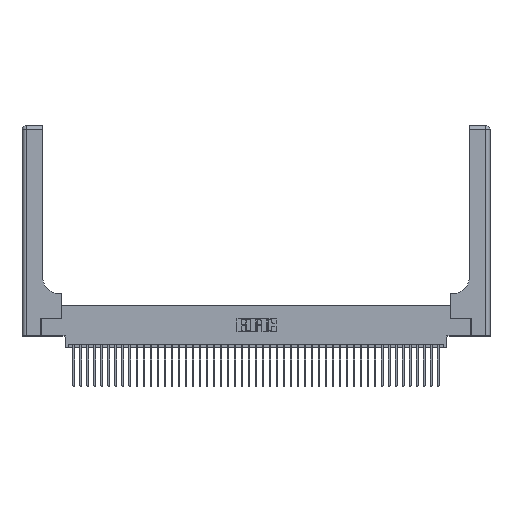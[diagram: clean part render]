
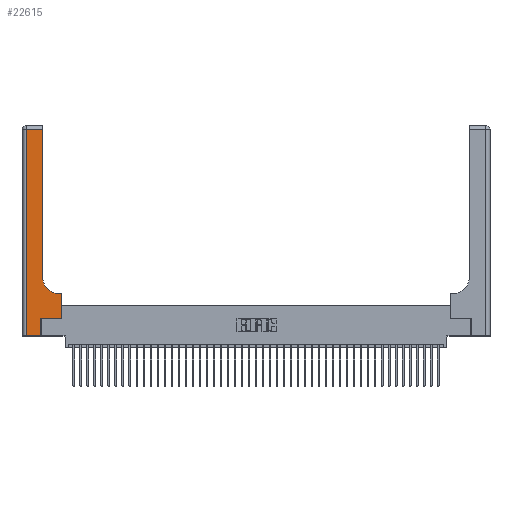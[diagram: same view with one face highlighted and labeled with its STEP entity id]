
A CAD part, top view. The second image highlights one B-rep face of the part: STEP entity #22615.
In plain terms, the highlighted planar face has unit normal (0, 0, 1).
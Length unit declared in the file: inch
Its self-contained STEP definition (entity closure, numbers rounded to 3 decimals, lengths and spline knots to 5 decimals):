
#1185 = VECTOR ( 'NONE', #26583, 39.37008 ) ;
#1284 = DIRECTION ( 'NONE',  ( 0., 1., 0. ) ) ;
#3033 = EDGE_LOOP ( 'NONE', ( #35671, #35020, #24982, #42316, #6401, #29921, #36176, #27049, #35757 ) ) ;
#3114 = VERTEX_POINT ( 'NONE', #22190 ) ;
#5375 = VECTOR ( 'NONE', #28450, 39.37008 ) ;
#5903 = VECTOR ( 'NONE', #1284, 39.37008 ) ;
#6401 = ORIENTED_EDGE ( 'NONE', *, *, #17791, .T. ) ;
#8280 = CARTESIAN_POINT ( 'NONE',  ( 0.5415, 0.6, 0.37 ) ) ;
#8372 = CARTESIAN_POINT ( 'NONE',  ( 0.2915, 0.6, 0.37 ) ) ;
#8870 = DIRECTION ( 'NONE',  ( 1., 0., 0. ) ) ;
#9039 = EDGE_CURVE ( 'NONE', #22875, #18721, #40002, .T. ) ;
#11078 = DIRECTION ( 'NONE',  ( 0., 0., -1. ) ) ;
#11527 = VERTEX_POINT ( 'NONE', #27741 ) ;
#11556 = CARTESIAN_POINT ( 'NONE',  ( 0.269, 0.25, 0.37 ) ) ;
#12474 = CARTESIAN_POINT ( 'NONE',  ( 0., 2.94, 0.37 ) ) ;
#12593 = VECTOR ( 'NONE', #8870, 39.37008 ) ;
#14444 = VERTEX_POINT ( 'NONE', #34162 ) ;
#15067 = CARTESIAN_POINT ( 'NONE',  ( 0.5415, 0.85, 0.37 ) ) ;
#16158 = DIRECTION ( 'NONE',  ( 0., -1., 0. ) ) ;
#16621 = VECTOR ( 'NONE', #16158, 39.37008 ) ;
#16697 = FACE_OUTER_BOUND ( 'NONE', #3033, .T. ) ;
#17165 = AXIS2_PLACEMENT_3D ( 'NONE', #20189, #44776, #23740 ) ;
#17302 = PLANE ( 'NONE',  #17165 ) ;
#17687 = LINE ( 'NONE', #23540, #39629 ) ;
#17791 = EDGE_CURVE ( 'NONE', #11527, #41406, #42154, .T. ) ;
#18196 = LINE ( 'NONE', #12474, #1185 ) ;
#18721 = VERTEX_POINT ( 'NONE', #8280 ) ;
#19135 = CARTESIAN_POINT ( 'NONE',  ( 0.269, 0.25, 0.37 ) ) ;
#20189 = CARTESIAN_POINT ( 'NONE',  ( 0., 3., 0.37 ) ) ;
#20246 = VERTEX_POINT ( 'NONE', #31881 ) ;
#20586 = LINE ( 'NONE', #45100, #38153 ) ;
#21670 = CARTESIAN_POINT ( 'NONE',  ( 0.06, 2.94, 0.37 ) ) ;
#21853 = EDGE_CURVE ( 'NONE', #20246, #14444, #20586, .T. ) ;
#22133 = CARTESIAN_POINT ( 'NONE',  ( 0.5585, 0.25, 0.37 ) ) ;
#22190 = CARTESIAN_POINT ( 'NONE',  ( 0.06, 0., 0.37 ) ) ;
#22615 = ADVANCED_FACE ( 'NONE', ( #16697 ), #17302, .F. ) ;
#22875 = VERTEX_POINT ( 'NONE', #31009 ) ;
#23358 = CIRCLE ( 'NONE', #31777, 0.25 ) ;
#23540 = CARTESIAN_POINT ( 'NONE',  ( 0., 0., 0.37 ) ) ;
#23740 = DIRECTION ( 'NONE',  ( -1., 0., 0. ) ) ;
#23902 = DIRECTION ( 'NONE',  ( 0., 1., 0. ) ) ;
#23905 = EDGE_CURVE ( 'NONE', #3114, #11527, #17687, .T. ) ;
#24695 = DIRECTION ( 'NONE',  ( -1., 0., 0. ) ) ;
#24982 = ORIENTED_EDGE ( 'NONE', *, *, #36821, .T. ) ;
#25312 = DIRECTION ( 'NONE',  ( 1., 0., 0. ) ) ;
#25450 = VERTEX_POINT ( 'NONE', #21670 ) ;
#25531 = EDGE_CURVE ( 'NONE', #31394, #22875, #40515, .T. ) ;
#26583 = DIRECTION ( 'NONE',  ( -1., 0., 0. ) ) ;
#27049 = ORIENTED_EDGE ( 'NONE', *, *, #9039, .T. ) ;
#27741 = CARTESIAN_POINT ( 'NONE',  ( 0.269, 0., 0.37 ) ) ;
#28450 = DIRECTION ( 'NONE',  ( 0., 1., 0. ) ) ;
#28769 = CARTESIAN_POINT ( 'NONE',  ( 0.269, 0., 0.37 ) ) ;
#29921 = ORIENTED_EDGE ( 'NONE', *, *, #43622, .T. ) ;
#30051 = CARTESIAN_POINT ( 'NONE',  ( 0.5585, 0.25, 0.37 ) ) ;
#31009 = CARTESIAN_POINT ( 'NONE',  ( 0.5585, 0.6, 0.37 ) ) ;
#31394 = VERTEX_POINT ( 'NONE', #30051 ) ;
#31777 = AXIS2_PLACEMENT_3D ( 'NONE', #15067, #11078, #25312 ) ;
#31881 = CARTESIAN_POINT ( 'NONE',  ( 0.2915, 0.85, 0.37 ) ) ;
#34162 = CARTESIAN_POINT ( 'NONE',  ( 0.2915, 2.94, 0.37 ) ) ;
#34482 = LINE ( 'NONE', #19135, #12593 ) ;
#35020 = ORIENTED_EDGE ( 'NONE', *, *, #41656, .T. ) ;
#35523 = EDGE_CURVE ( 'NONE', #18721, #20246, #23358, .T. ) ;
#35671 = ORIENTED_EDGE ( 'NONE', *, *, #21853, .T. ) ;
#35757 = ORIENTED_EDGE ( 'NONE', *, *, #35523, .T. ) ;
#36176 = ORIENTED_EDGE ( 'NONE', *, *, #25531, .T. ) ;
#36821 = EDGE_CURVE ( 'NONE', #25450, #3114, #43528, .T. ) ;
#38153 = VECTOR ( 'NONE', #23902, 39.37008 ) ;
#39629 = VECTOR ( 'NONE', #44263, 39.37008 ) ;
#40002 = LINE ( 'NONE', #8372, #43882 ) ;
#40515 = LINE ( 'NONE', #22133, #5375 ) ;
#40861 = CARTESIAN_POINT ( 'NONE',  ( 0.06, 3., 0.37 ) ) ;
#41406 = VERTEX_POINT ( 'NONE', #11556 ) ;
#41656 = EDGE_CURVE ( 'NONE', #14444, #25450, #18196, .T. ) ;
#42154 = LINE ( 'NONE', #28769, #5903 ) ;
#42316 = ORIENTED_EDGE ( 'NONE', *, *, #23905, .T. ) ;
#43528 = LINE ( 'NONE', #40861, #16621 ) ;
#43622 = EDGE_CURVE ( 'NONE', #41406, #31394, #34482, .T. ) ;
#43882 = VECTOR ( 'NONE', #24695, 39.37008 ) ;
#44263 = DIRECTION ( 'NONE',  ( 1., 0., 0. ) ) ;
#44776 = DIRECTION ( 'NONE',  ( 0., 0., -1. ) ) ;
#45100 = CARTESIAN_POINT ( 'NONE',  ( 0.2915, 3., 0.37 ) ) ;
